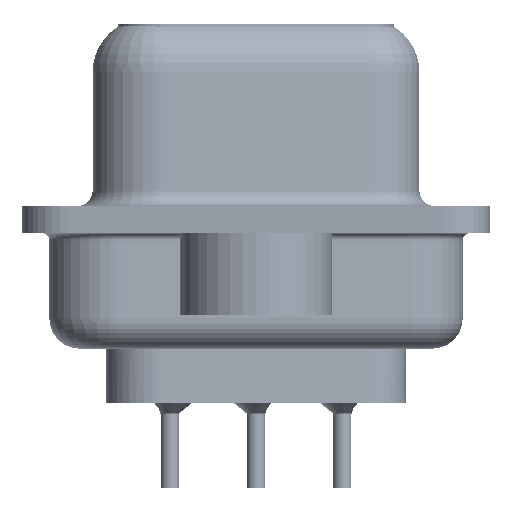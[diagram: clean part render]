
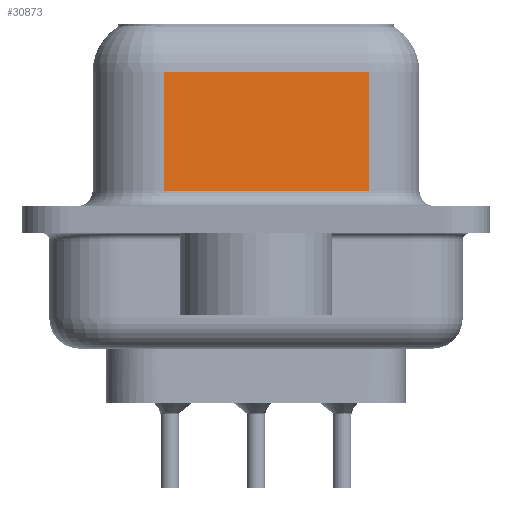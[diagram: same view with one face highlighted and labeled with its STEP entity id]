
A CAD part, left-side view. The second image highlights one B-rep face of the part: STEP entity #30873.
In plain terms, the highlighted planar face has unit normal (-0.985, -0.174, 0).
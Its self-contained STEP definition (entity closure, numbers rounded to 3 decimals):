
#112 = EDGE_LOOP ( 'NONE', ( #22647, #26359, #12918, #6895 ) ) ;
#880 = LINE ( 'NONE', #23992, #7453 ) ;
#1140 = EDGE_CURVE ( 'NONE', #31252, #2448, #33352, .T. ) ;
#2448 = VERTEX_POINT ( 'NONE', #9109 ) ;
#4718 = DIRECTION ( 'NONE',  ( 0., 0., -1. ) ) ;
#5438 = CARTESIAN_POINT ( 'NONE',  ( 5.621, -3.722, 0.95 ) ) ;
#5818 = CARTESIAN_POINT ( 'NONE',  ( 5.621, -3.722, 0.95 ) ) ;
#6728 = EDGE_CURVE ( 'NONE', #10987, #31252, #24954, .T. ) ;
#6792 = PLANE ( 'NONE',  #28725 ) ;
#6895 = ORIENTED_EDGE ( 'NONE', *, *, #32315, .T. ) ;
#7453 = VECTOR ( 'NONE', #4718, 1000. ) ;
#7684 = CARTESIAN_POINT ( 'NONE',  ( 5.621, -3.722, 4.85 ) ) ;
#7884 = CARTESIAN_POINT ( 'NONE',  ( 5.621, -3.722, 4.85 ) ) ;
#9109 = CARTESIAN_POINT ( 'NONE',  ( 4.43, 3.028, 0.95 ) ) ;
#9810 = DIRECTION ( 'NONE',  ( 0., 0., -1. ) ) ;
#9816 = CARTESIAN_POINT ( 'NONE',  ( 5.621, -3.722, 6.6 ) ) ;
#9924 = CARTESIAN_POINT ( 'NONE',  ( 4.43, 3.028, 4.85 ) ) ;
#9956 = DIRECTION ( 'NONE',  ( -0.174, 0.985, 0. ) ) ;
#10987 = VERTEX_POINT ( 'NONE', #7884 ) ;
#12176 = CARTESIAN_POINT ( 'NONE',  ( 4.43, 3.028, 6.6 ) ) ;
#12794 = EDGE_CURVE ( 'NONE', #10987, #25874, #880, .T. ) ;
#12918 = ORIENTED_EDGE ( 'NONE', *, *, #1140, .T. ) ;
#14031 = DIRECTION ( 'NONE',  ( -0.174, 0.985, 0. ) ) ;
#18543 = FACE_OUTER_BOUND ( 'NONE', #112, .T. ) ;
#22437 = LINE ( 'NONE', #5818, #39647 ) ;
#22647 = ORIENTED_EDGE ( 'NONE', *, *, #12794, .F. ) ;
#23992 = CARTESIAN_POINT ( 'NONE',  ( 5.621, -3.722, 6.6 ) ) ;
#24954 = LINE ( 'NONE', #7684, #41150 ) ;
#25874 = VERTEX_POINT ( 'NONE', #5438 ) ;
#26299 = DIRECTION ( 'NONE',  ( 0.174, -0.985, 0. ) ) ;
#26359 = ORIENTED_EDGE ( 'NONE', *, *, #6728, .T. ) ;
#28725 = AXIS2_PLACEMENT_3D ( 'NONE', #9816, #29353, #9956 ) ;
#29353 = DIRECTION ( 'NONE',  ( 0.985, 0.174, 0. ) ) ;
#30873 = ADVANCED_FACE ( 'NONE', ( #18543 ), #6792, .F. ) ;
#31252 = VERTEX_POINT ( 'NONE', #9924 ) ;
#32315 = EDGE_CURVE ( 'NONE', #2448, #25874, #22437, .T. ) ;
#33352 = LINE ( 'NONE', #12176, #39887 ) ;
#39647 = VECTOR ( 'NONE', #26299, 1000. ) ;
#39887 = VECTOR ( 'NONE', #9810, 1000. ) ;
#41150 = VECTOR ( 'NONE', #14031, 1000. ) ;
